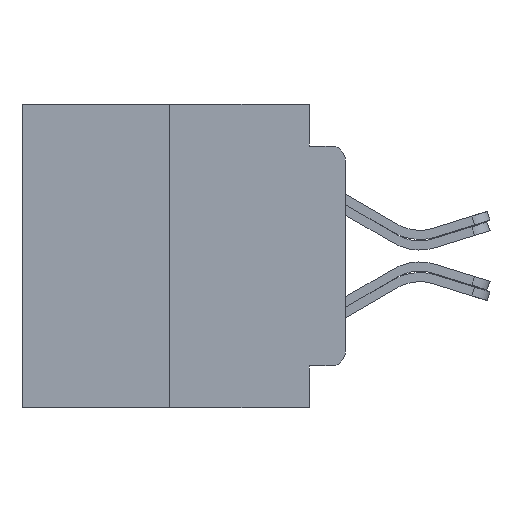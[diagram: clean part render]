
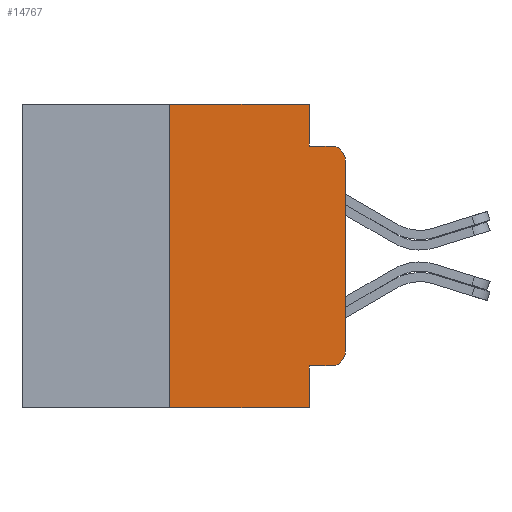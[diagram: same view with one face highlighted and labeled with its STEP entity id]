
A CAD part, left-side view. The second image highlights one B-rep face of the part: STEP entity #14767.
In plain terms, the highlighted planar face has unit normal (-1, 0, 0).
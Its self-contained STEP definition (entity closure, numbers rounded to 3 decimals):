
#162 = CARTESIAN_POINT ( 'NONE',  ( -75.603, 1.295, 0. ) ) ;
#167 = CARTESIAN_POINT ( 'NONE',  ( -75.603, 0., 3.467 ) ) ;
#587 = EDGE_CURVE ( 'NONE', #8868, #818, #21863, .T. ) ;
#751 = EDGE_CURVE ( 'NONE', #14827, #11731, #28457, .T. ) ;
#794 = EDGE_CURVE ( 'NONE', #8728, #10915, #5251, .T. ) ;
#818 = VERTEX_POINT ( 'NONE', #7718 ) ;
#1608 = EDGE_CURVE ( 'NONE', #27897, #2081, #18037, .T. ) ;
#2081 = VERTEX_POINT ( 'NONE', #167 ) ;
#2107 = CARTESIAN_POINT ( 'NONE',  ( -75.603, 1.295, 3.975 ) ) ;
#2533 = VECTOR ( 'NONE', #27901, 1000. ) ;
#3072 = DIRECTION ( 'NONE',  ( 0., -1., 0. ) ) ;
#5251 = LINE ( 'NONE', #16570, #5934 ) ;
#5373 = CARTESIAN_POINT ( 'NONE',  ( -75.603, 0.508, 3.975 ) ) ;
#5386 = DIRECTION ( 'NONE',  ( 0., 0., -1. ) ) ;
#5416 = DIRECTION ( 'NONE',  ( 0., -1., 0. ) ) ;
#5934 = VECTOR ( 'NONE', #5386, 1000. ) ;
#6020 = EDGE_CURVE ( 'NONE', #8868, #11731, #27237, .T. ) ;
#6102 = VECTOR ( 'NONE', #22786, 1000. ) ;
#6288 = VECTOR ( 'NONE', #18153, 1000. ) ;
#6734 = CARTESIAN_POINT ( 'NONE',  ( -75.603, 0.508, -3.467 ) ) ;
#6887 = DIRECTION ( 'NONE',  ( 0., 0., -1. ) ) ;
#7229 = CARTESIAN_POINT ( 'NONE',  ( -75.603, 0., 5.486 ) ) ;
#7281 = ORIENTED_EDGE ( 'NONE', *, *, #794, .F. ) ;
#7718 = CARTESIAN_POINT ( 'NONE',  ( -75.603, 6.35, 5.486 ) ) ;
#8043 = DIRECTION ( 'NONE',  ( 1., 0., 0. ) ) ;
#8081 = AXIS2_PLACEMENT_3D ( 'NONE', #21178, #27575, #18991 ) ;
#8648 = AXIS2_PLACEMENT_3D ( 'NONE', #6734, #15539, #21900 ) ;
#8728 = VERTEX_POINT ( 'NONE', #19028 ) ;
#8868 = VERTEX_POINT ( 'NONE', #22809 ) ;
#9888 = LINE ( 'NONE', #18680, #11281 ) ;
#9988 = LINE ( 'NONE', #16371, #18294 ) ;
#10157 = ORIENTED_EDGE ( 'NONE', *, *, #20775, .F. ) ;
#10255 = EDGE_LOOP ( 'NONE', ( #14331, #14098, #23879, #10560, #15554, #7281, #10157, #13200, #16495, #17808 ) ) ;
#10396 = VERTEX_POINT ( 'NONE', #15718 ) ;
#10560 = ORIENTED_EDGE ( 'NONE', *, *, #17329, .T. ) ;
#10785 = DIRECTION ( 'NONE',  ( 0., 0., 1. ) ) ;
#10915 = VERTEX_POINT ( 'NONE', #2107 ) ;
#11281 = VECTOR ( 'NONE', #5416, 1000. ) ;
#11293 = AXIS2_PLACEMENT_3D ( 'NONE', #23670, #8043, #14811 ) ;
#11731 = VERTEX_POINT ( 'NONE', #14653 ) ;
#12404 = PLANE ( 'NONE',  #11293 ) ;
#13200 = ORIENTED_EDGE ( 'NONE', *, *, #587, .F. ) ;
#13738 = EDGE_CURVE ( 'NONE', #10396, #27897, #23597, .T. ) ;
#14098 = ORIENTED_EDGE ( 'NONE', *, *, #13738, .T. ) ;
#14331 = ORIENTED_EDGE ( 'NONE', *, *, #20241, .T. ) ;
#14653 = CARTESIAN_POINT ( 'NONE',  ( -75.603, 1.295, -5.486 ) ) ;
#14767 = ADVANCED_FACE ( 'NONE', ( #15608 ), #12404, .F. ) ;
#14811 = DIRECTION ( 'NONE',  ( 0., 0., -1. ) ) ;
#14827 = VERTEX_POINT ( 'NONE', #14898 ) ;
#14898 = CARTESIAN_POINT ( 'NONE',  ( -75.603, 1.295, -3.975 ) ) ;
#15539 = DIRECTION ( 'NONE',  ( -1., 0., 0. ) ) ;
#15554 = ORIENTED_EDGE ( 'NONE', *, *, #26798, .F. ) ;
#15608 = FACE_OUTER_BOUND ( 'NONE', #10255, .T. ) ;
#15718 = CARTESIAN_POINT ( 'NONE',  ( -75.603, 0.508, -3.975 ) ) ;
#16371 = CARTESIAN_POINT ( 'NONE',  ( -75.603, 1.295, -3.975 ) ) ;
#16495 = ORIENTED_EDGE ( 'NONE', *, *, #6020, .T. ) ;
#16570 = CARTESIAN_POINT ( 'NONE',  ( -75.603, 1.295, 0. ) ) ;
#17329 = EDGE_CURVE ( 'NONE', #2081, #19051, #25821, .T. ) ;
#17808 = ORIENTED_EDGE ( 'NONE', *, *, #751, .F. ) ;
#18037 = LINE ( 'NONE', #7229, #6288 ) ;
#18153 = DIRECTION ( 'NONE',  ( 0., 0., 1. ) ) ;
#18294 = VECTOR ( 'NONE', #3072, 1000. ) ;
#18680 = CARTESIAN_POINT ( 'NONE',  ( -75.603, 1.295, 3.975 ) ) ;
#18991 = DIRECTION ( 'NONE',  ( 0., 0., -1. ) ) ;
#19028 = CARTESIAN_POINT ( 'NONE',  ( -75.603, 1.295, 5.486 ) ) ;
#19051 = VERTEX_POINT ( 'NONE', #5373 ) ;
#20241 = EDGE_CURVE ( 'NONE', #14827, #10396, #9988, .T. ) ;
#20274 = CARTESIAN_POINT ( 'NONE',  ( -75.603, 0., -3.467 ) ) ;
#20775 = EDGE_CURVE ( 'NONE', #818, #8728, #21659, .T. ) ;
#21178 = CARTESIAN_POINT ( 'NONE',  ( -75.603, 0.508, 3.467 ) ) ;
#21659 = LINE ( 'NONE', #22689, #6102 ) ;
#21863 = LINE ( 'NONE', #21955, #26720 ) ;
#21900 = DIRECTION ( 'NONE',  ( 0., 0., -1. ) ) ;
#21955 = CARTESIAN_POINT ( 'NONE',  ( -75.603, 6.35, -5.486 ) ) ;
#22556 = VECTOR ( 'NONE', #6887, 1000. ) ;
#22689 = CARTESIAN_POINT ( 'NONE',  ( -75.603, 11.684, 5.486 ) ) ;
#22786 = DIRECTION ( 'NONE',  ( 0., -1., 0. ) ) ;
#22809 = CARTESIAN_POINT ( 'NONE',  ( -75.603, 6.35, -5.486 ) ) ;
#23597 = CIRCLE ( 'NONE', #8648, 0.508 ) ;
#23670 = CARTESIAN_POINT ( 'NONE',  ( -75.603, 11.684, 5.486 ) ) ;
#23879 = ORIENTED_EDGE ( 'NONE', *, *, #1608, .T. ) ;
#25821 = CIRCLE ( 'NONE', #8081, 0.508 ) ;
#26720 = VECTOR ( 'NONE', #10785, 1000. ) ;
#26798 = EDGE_CURVE ( 'NONE', #10915, #19051, #9888, .T. ) ;
#27237 = LINE ( 'NONE', #28003, #2533 ) ;
#27575 = DIRECTION ( 'NONE',  ( -1., 0., 0. ) ) ;
#27897 = VERTEX_POINT ( 'NONE', #20274 ) ;
#27901 = DIRECTION ( 'NONE',  ( 0., -1., 0. ) ) ;
#28003 = CARTESIAN_POINT ( 'NONE',  ( -75.603, 11.684, -5.486 ) ) ;
#28457 = LINE ( 'NONE', #162, #22556 ) ;
